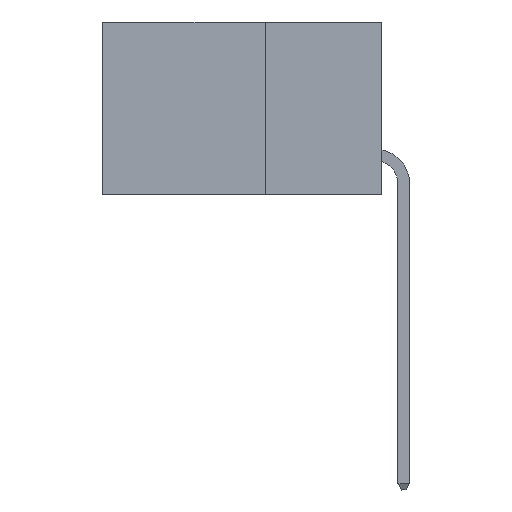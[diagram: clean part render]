
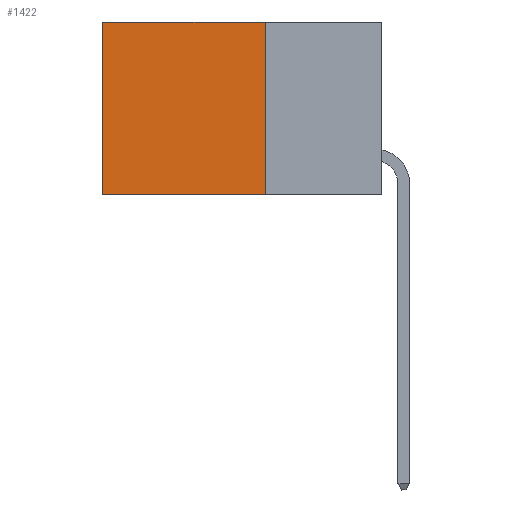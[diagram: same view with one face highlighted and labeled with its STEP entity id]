
A CAD part, left-side view. The second image highlights one B-rep face of the part: STEP entity #1422.
In plain terms, the highlighted planar face has unit normal (-1, 0, 0).
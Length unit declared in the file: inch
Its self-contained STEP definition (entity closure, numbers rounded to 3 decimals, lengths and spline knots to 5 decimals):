
#13 = ORIENTED_EDGE ( 'NONE', *, *, #11998, .F. ) ;
#96 = VECTOR ( 'NONE', #3035, 39.37008 ) ;
#428 = LINE ( 'NONE', #5063, #849 ) ;
#849 = VECTOR ( 'NONE', #14481, 39.37008 ) ;
#1422 = ADVANCED_FACE ( 'NONE', ( #10651 ), #16661, .F. ) ;
#3035 = DIRECTION ( 'NONE',  ( 0., 1., 0. ) ) ;
#3251 = CARTESIAN_POINT ( 'NONE',  ( 0.2875, 0.25, -0.37 ) ) ;
#3683 = CARTESIAN_POINT ( 'NONE',  ( 0.2875, 0.25, -0.37 ) ) ;
#4079 = VERTEX_POINT ( 'NONE', #12824 ) ;
#4421 = VECTOR ( 'NONE', #14345, 39.37008 ) ;
#4824 = EDGE_CURVE ( 'NONE', #6896, #4079, #12145, .T. ) ;
#5063 = CARTESIAN_POINT ( 'NONE',  ( 0.2875, 0.25, 0. ) ) ;
#6179 = CARTESIAN_POINT ( 'NONE',  ( 0.2875, 0.6, 0. ) ) ;
#6852 = VERTEX_POINT ( 'NONE', #11008 ) ;
#6896 = VERTEX_POINT ( 'NONE', #15804 ) ;
#7144 = CARTESIAN_POINT ( 'NONE',  ( 0.2875, 0.25, 0. ) ) ;
#7580 = EDGE_CURVE ( 'NONE', #4079, #6852, #8030, .T. ) ;
#7641 = LINE ( 'NONE', #3251, #96 ) ;
#8030 = LINE ( 'NONE', #6179, #4421 ) ;
#8287 = EDGE_CURVE ( 'NONE', #6896, #10533, #428, .T. ) ;
#8295 = ORIENTED_EDGE ( 'NONE', *, *, #7580, .T. ) ;
#8423 = DIRECTION ( 'NONE',  ( 1., 0., 0. ) ) ;
#8824 = AXIS2_PLACEMENT_3D ( 'NONE', #7144, #8423, #15138 ) ;
#10533 = VERTEX_POINT ( 'NONE', #3683 ) ;
#10651 = FACE_OUTER_BOUND ( 'NONE', #11747, .T. ) ;
#11008 = CARTESIAN_POINT ( 'NONE',  ( 0.2875, 0.6, -0.37 ) ) ;
#11117 = VECTOR ( 'NONE', #16851, 39.37008 ) ;
#11747 = EDGE_LOOP ( 'NONE', ( #8295, #13, #13604, #15412 ) ) ;
#11998 = EDGE_CURVE ( 'NONE', #10533, #6852, #7641, .T. ) ;
#12145 = LINE ( 'NONE', #15515, #11117 ) ;
#12824 = CARTESIAN_POINT ( 'NONE',  ( 0.2875, 0.6, 0. ) ) ;
#13604 = ORIENTED_EDGE ( 'NONE', *, *, #8287, .F. ) ;
#14345 = DIRECTION ( 'NONE',  ( 0., 0., -1. ) ) ;
#14481 = DIRECTION ( 'NONE',  ( 0., 0., -1. ) ) ;
#15138 = DIRECTION ( 'NONE',  ( 0., 0., -1. ) ) ;
#15412 = ORIENTED_EDGE ( 'NONE', *, *, #4824, .T. ) ;
#15515 = CARTESIAN_POINT ( 'NONE',  ( 0.2875, 0.25, 0. ) ) ;
#15804 = CARTESIAN_POINT ( 'NONE',  ( 0.2875, 0.25, 0. ) ) ;
#16661 = PLANE ( 'NONE',  #8824 ) ;
#16851 = DIRECTION ( 'NONE',  ( 0., 1., 0. ) ) ;
